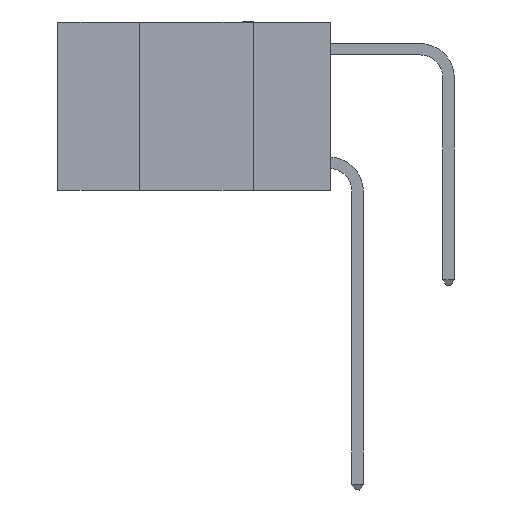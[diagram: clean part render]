
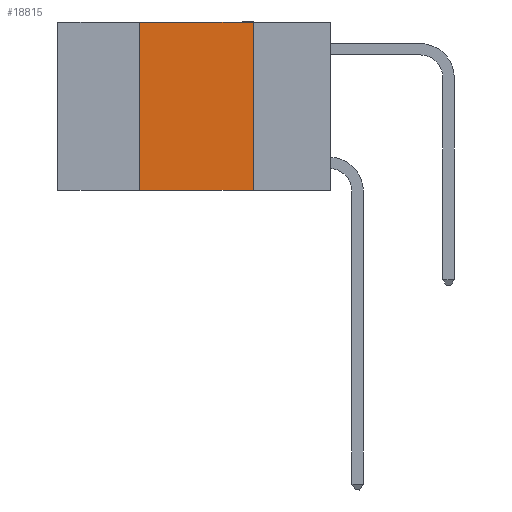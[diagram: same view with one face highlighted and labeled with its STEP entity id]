
A CAD part, left-side view. The second image highlights one B-rep face of the part: STEP entity #18815.
In plain terms, the highlighted planar face has unit normal (-1, 0, 0).
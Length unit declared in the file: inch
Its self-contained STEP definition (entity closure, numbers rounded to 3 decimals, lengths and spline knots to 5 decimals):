
#548 = VECTOR ( 'NONE', #5911, 39.37008 ) ;
#1260 = CARTESIAN_POINT ( 'NONE',  ( 0., 0.6, 0. ) ) ;
#1837 = DIRECTION ( 'NONE',  ( 0., 0., 1. ) ) ;
#1997 = VECTOR ( 'NONE', #3173, 39.37008 ) ;
#3173 = DIRECTION ( 'NONE',  ( 0., -1., 0. ) ) ;
#3492 = ORIENTED_EDGE ( 'NONE', *, *, #18256, .T. ) ;
#3707 = PLANE ( 'NONE',  #14202 ) ;
#5793 = CARTESIAN_POINT ( 'NONE',  ( 0., 0.17, 0. ) ) ;
#5911 = DIRECTION ( 'NONE',  ( 0., -1., 0. ) ) ;
#6360 = ORIENTED_EDGE ( 'NONE', *, *, #21965, .F. ) ;
#7413 = DIRECTION ( 'NONE',  ( 0., 0., -1. ) ) ;
#8208 = CARTESIAN_POINT ( 'NONE',  ( 0., 0.17, -0.37 ) ) ;
#8723 = LINE ( 'NONE', #5793, #23145 ) ;
#9629 = CARTESIAN_POINT ( 'NONE',  ( 0., 0.42, -0.37 ) ) ;
#10104 = EDGE_CURVE ( 'NONE', #20464, #12579, #8723, .T. ) ;
#10448 = LINE ( 'NONE', #13241, #548 ) ;
#11071 = CARTESIAN_POINT ( 'NONE',  ( 0., 0.42, 0. ) ) ;
#11149 = EDGE_CURVE ( 'NONE', #11518, #20464, #11830, .T. ) ;
#11518 = VERTEX_POINT ( 'NONE', #16947 ) ;
#11830 = LINE ( 'NONE', #1260, #1997 ) ;
#12579 = VERTEX_POINT ( 'NONE', #8208 ) ;
#13241 = CARTESIAN_POINT ( 'NONE',  ( 0., 0.6, -0.37 ) ) ;
#14132 = EDGE_LOOP ( 'NONE', ( #15536, #19775, #6360, #3492 ) ) ;
#14202 = AXIS2_PLACEMENT_3D ( 'NONE', #16535, #18373, #7413 ) ;
#15536 = ORIENTED_EDGE ( 'NONE', *, *, #10104, .F. ) ;
#16535 = CARTESIAN_POINT ( 'NONE',  ( 0., 0.6, 0. ) ) ;
#16947 = CARTESIAN_POINT ( 'NONE',  ( 0., 0.42, 0. ) ) ;
#18256 = EDGE_CURVE ( 'NONE', #18261, #12579, #10448, .T. ) ;
#18261 = VERTEX_POINT ( 'NONE', #9629 ) ;
#18373 = DIRECTION ( 'NONE',  ( 1., 0., 0. ) ) ;
#18594 = DIRECTION ( 'NONE',  ( 0., 0., -1. ) ) ;
#18815 = ADVANCED_FACE ( 'NONE', ( #22881 ), #3707, .F. ) ;
#19775 = ORIENTED_EDGE ( 'NONE', *, *, #11149, .F. ) ;
#20464 = VERTEX_POINT ( 'NONE', #20874 ) ;
#20874 = CARTESIAN_POINT ( 'NONE',  ( 0., 0.17, 0. ) ) ;
#21603 = VECTOR ( 'NONE', #1837, 39.37008 ) ;
#21965 = EDGE_CURVE ( 'NONE', #18261, #11518, #22158, .T. ) ;
#22158 = LINE ( 'NONE', #11071, #21603 ) ;
#22881 = FACE_OUTER_BOUND ( 'NONE', #14132, .T. ) ;
#23145 = VECTOR ( 'NONE', #18594, 39.37008 ) ;
